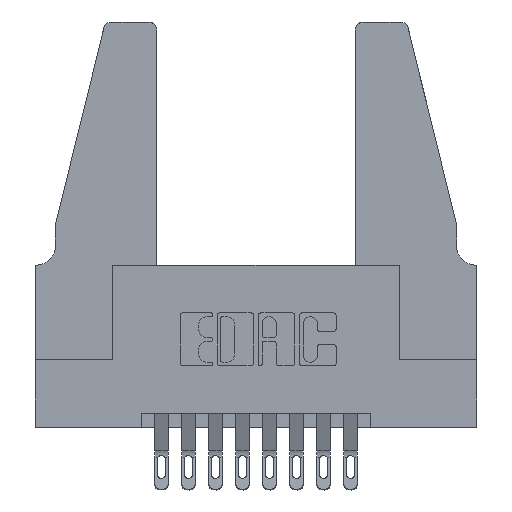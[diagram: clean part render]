
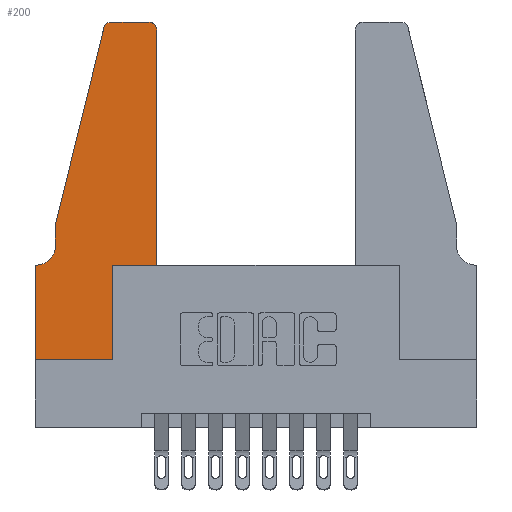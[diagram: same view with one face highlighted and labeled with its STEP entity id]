
A CAD part, top view. The second image highlights one B-rep face of the part: STEP entity #200.
In plain terms, the highlighted planar face has unit normal (0, 0, 1).
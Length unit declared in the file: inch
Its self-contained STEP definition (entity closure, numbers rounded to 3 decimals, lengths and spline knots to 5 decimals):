
#42 = AXIS2_PLACEMENT_3D ( 'NONE', #1760, #869, #11048 ) ;
#200 = ADVANCED_FACE ( 'NONE', ( #1471 ), #9601, .T. ) ;
#504 = ORIENTED_EDGE ( 'NONE', *, *, #3674, .T. ) ;
#683 = CARTESIAN_POINT ( 'NONE',  ( 0.0755, 0.42, 0.37 ) ) ;
#689 = CARTESIAN_POINT ( 'NONE',  ( 0., 0., 0.37 ) ) ;
#826 = CARTESIAN_POINT ( 'NONE',  ( 0.284, 1.25, 0.37 ) ) ;
#830 = VECTOR ( 'NONE', #12764, 39.37008 ) ;
#849 = EDGE_CURVE ( 'NONE', #3451, #5381, #9370, .T. ) ;
#869 = DIRECTION ( 'NONE',  ( 0., 0., 1. ) ) ;
#963 = LINE ( 'NONE', #4086, #4641 ) ;
#1048 = EDGE_LOOP ( 'NONE', ( #3355, #1720, #3098, #1435, #8142, #10184, #11293, #12356, #2061, #5298, #6803, #504 ) ) ;
#1239 = LINE ( 'NONE', #7240, #10898 ) ;
#1278 = LINE ( 'NONE', #7038, #2888 ) ;
#1435 = ORIENTED_EDGE ( 'NONE', *, *, #5765, .T. ) ;
#1449 = DIRECTION ( 'NONE',  ( 1., 0., 0. ) ) ;
#1471 = FACE_OUTER_BOUND ( 'NONE', #1048, .T. ) ;
#1586 = EDGE_CURVE ( 'NONE', #1724, #2698, #1278, .T. ) ;
#1637 = LINE ( 'NONE', #2376, #10828 ) ;
#1697 = CARTESIAN_POINT ( 'NONE',  ( 0.0755, 0.5, 0.37 ) ) ;
#1720 = ORIENTED_EDGE ( 'NONE', *, *, #11777, .T. ) ;
#1724 = VERTEX_POINT ( 'NONE', #5216 ) ;
#1760 = CARTESIAN_POINT ( 'NONE',  ( 0.4205, 1.22, 0.37 ) ) ;
#1813 = EDGE_CURVE ( 'NONE', #12384, #11979, #963, .T. ) ;
#1830 = LINE ( 'NONE', #6516, #4213 ) ;
#1921 = LINE ( 'NONE', #689, #9963 ) ;
#2019 = EDGE_CURVE ( 'NONE', #4118, #6446, #1921, .T. ) ;
#2061 = ORIENTED_EDGE ( 'NONE', *, *, #9777, .T. ) ;
#2340 = VERTEX_POINT ( 'NONE', #11745 ) ;
#2376 = CARTESIAN_POINT ( 'NONE',  ( 0., 0., 0.37 ) ) ;
#2424 = DIRECTION ( 'NONE',  ( 0., -1., 0. ) ) ;
#2569 = DIRECTION ( 'NONE',  ( 1., 0., 0. ) ) ;
#2698 = VERTEX_POINT ( 'NONE', #3221 ) ;
#2723 = EDGE_CURVE ( 'NONE', #5652, #1724, #10105, .T. ) ;
#2740 = DIRECTION ( 'NONE',  ( -0.239, -0.971, 0. ) ) ;
#2888 = VECTOR ( 'NONE', #13275, 39.37008 ) ;
#3069 = CARTESIAN_POINT ( 'NONE',  ( 0.4205, 1.25, 0.37 ) ) ;
#3098 = ORIENTED_EDGE ( 'NONE', *, *, #3284, .T. ) ;
#3221 = CARTESIAN_POINT ( 'NONE',  ( 0., 0.35, 0.37 ) ) ;
#3284 = EDGE_CURVE ( 'NONE', #5794, #2340, #12530, .T. ) ;
#3334 = CIRCLE ( 'NONE', #42, 0.03 ) ;
#3355 = ORIENTED_EDGE ( 'NONE', *, *, #849, .T. ) ;
#3451 = VERTEX_POINT ( 'NONE', #3069 ) ;
#3519 = AXIS2_PLACEMENT_3D ( 'NONE', #12777, #7646, #1449 ) ;
#3674 = EDGE_CURVE ( 'NONE', #11979, #3451, #3334, .T. ) ;
#4086 = CARTESIAN_POINT ( 'NONE',  ( 0.4505, 0.35, 0.37 ) ) ;
#4118 = VERTEX_POINT ( 'NONE', #4488 ) ;
#4163 = LINE ( 'NONE', #5987, #8864 ) ;
#4213 = VECTOR ( 'NONE', #11766, 39.37008 ) ;
#4274 = CARTESIAN_POINT ( 'NONE',  ( 0.25487, 1.22718, 0.37 ) ) ;
#4488 = CARTESIAN_POINT ( 'NONE',  ( 0., 0., 0.37 ) ) ;
#4590 = DIRECTION ( 'NONE',  ( -1., 0., 0. ) ) ;
#4641 = VECTOR ( 'NONE', #6197, 39.37008 ) ;
#4671 = DIRECTION ( 'NONE',  ( 0., 0., -1. ) ) ;
#5026 = AXIS2_PLACEMENT_3D ( 'NONE', #10772, #4671, #4590 ) ;
#5216 = CARTESIAN_POINT ( 'NONE',  ( 0.0055, 0.35, 0.37 ) ) ;
#5298 = ORIENTED_EDGE ( 'NONE', *, *, #11201, .T. ) ;
#5381 = VERTEX_POINT ( 'NONE', #826 ) ;
#5592 = CARTESIAN_POINT ( 'NONE',  ( 0.4505, 0.35, 0.37 ) ) ;
#5652 = VERTEX_POINT ( 'NONE', #683 ) ;
#5765 = EDGE_CURVE ( 'NONE', #2340, #5652, #1239, .T. ) ;
#5794 = VERTEX_POINT ( 'NONE', #4274 ) ;
#5987 = CARTESIAN_POINT ( 'NONE',  ( 0.2865, 0.35, 0.37 ) ) ;
#6075 = CARTESIAN_POINT ( 'NONE',  ( 0.4505, 1.22, 0.37 ) ) ;
#6197 = DIRECTION ( 'NONE',  ( 0., 1., 0. ) ) ;
#6446 = VERTEX_POINT ( 'NONE', #12814 ) ;
#6468 = DIRECTION ( 'NONE',  ( 1., 0., 0. ) ) ;
#6516 = CARTESIAN_POINT ( 'NONE',  ( 0.4505, 0.35, 0.37 ) ) ;
#6803 = ORIENTED_EDGE ( 'NONE', *, *, #1813, .T. ) ;
#6835 = AXIS2_PLACEMENT_3D ( 'NONE', #7720, #8736, #2569 ) ;
#7038 = CARTESIAN_POINT ( 'NONE',  ( 0.0755, 0.35, 0.37 ) ) ;
#7240 = CARTESIAN_POINT ( 'NONE',  ( 0.0755, 0.5, 0.37 ) ) ;
#7646 = DIRECTION ( 'NONE',  ( 0., 0., 1. ) ) ;
#7720 = CARTESIAN_POINT ( 'NONE',  ( 0.284, 1.22, 0.37 ) ) ;
#8124 = CIRCLE ( 'NONE', #6835, 0.03 ) ;
#8142 = ORIENTED_EDGE ( 'NONE', *, *, #2723, .T. ) ;
#8521 = CARTESIAN_POINT ( 'NONE',  ( 0.2605, 1.25, 0.37 ) ) ;
#8668 = VECTOR ( 'NONE', #2740, 39.37008 ) ;
#8736 = DIRECTION ( 'NONE',  ( 0., 0., 1. ) ) ;
#8864 = VECTOR ( 'NONE', #12194, 39.37008 ) ;
#9370 = LINE ( 'NONE', #8521, #830 ) ;
#9601 = PLANE ( 'NONE',  #3519 ) ;
#9777 = EDGE_CURVE ( 'NONE', #6446, #11320, #4163, .T. ) ;
#9963 = VECTOR ( 'NONE', #6468, 39.37008 ) ;
#10105 = CIRCLE ( 'NONE', #5026, 0.07 ) ;
#10184 = ORIENTED_EDGE ( 'NONE', *, *, #1586, .T. ) ;
#10237 = CARTESIAN_POINT ( 'NONE',  ( 0.2865, 0.35, 0.37 ) ) ;
#10772 = CARTESIAN_POINT ( 'NONE',  ( 0.0055, 0.42, 0.37 ) ) ;
#10828 = VECTOR ( 'NONE', #2424, 39.37008 ) ;
#10898 = VECTOR ( 'NONE', #13327, 39.37008 ) ;
#11048 = DIRECTION ( 'NONE',  ( 1., 0., 0. ) ) ;
#11201 = EDGE_CURVE ( 'NONE', #11320, #12384, #1830, .T. ) ;
#11293 = ORIENTED_EDGE ( 'NONE', *, *, #12957, .T. ) ;
#11320 = VERTEX_POINT ( 'NONE', #10237 ) ;
#11745 = CARTESIAN_POINT ( 'NONE',  ( 0.0755, 0.5, 0.37 ) ) ;
#11766 = DIRECTION ( 'NONE',  ( 1., 0., 0. ) ) ;
#11777 = EDGE_CURVE ( 'NONE', #5381, #5794, #8124, .T. ) ;
#11979 = VERTEX_POINT ( 'NONE', #6075 ) ;
#12194 = DIRECTION ( 'NONE',  ( 0., 1., 0. ) ) ;
#12356 = ORIENTED_EDGE ( 'NONE', *, *, #2019, .T. ) ;
#12384 = VERTEX_POINT ( 'NONE', #5592 ) ;
#12530 = LINE ( 'NONE', #1697, #8668 ) ;
#12764 = DIRECTION ( 'NONE',  ( -1., 0., 0. ) ) ;
#12777 = CARTESIAN_POINT ( 'NONE',  ( 0., 0.35, 0.37 ) ) ;
#12814 = CARTESIAN_POINT ( 'NONE',  ( 0.2865, 0., 0.37 ) ) ;
#12957 = EDGE_CURVE ( 'NONE', #2698, #4118, #1637, .T. ) ;
#13275 = DIRECTION ( 'NONE',  ( -1., 0., 0. ) ) ;
#13327 = DIRECTION ( 'NONE',  ( 0., -1., 0. ) ) ;
